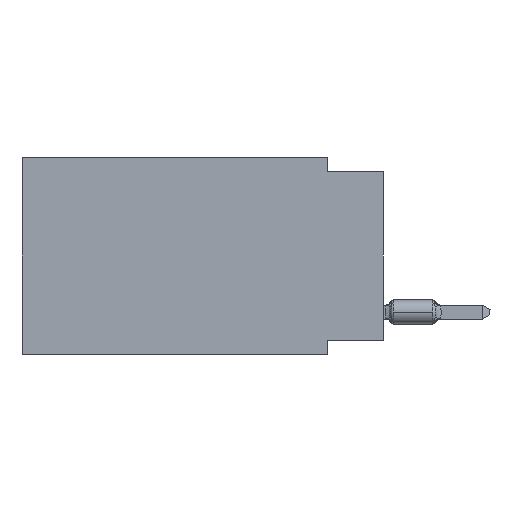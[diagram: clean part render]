
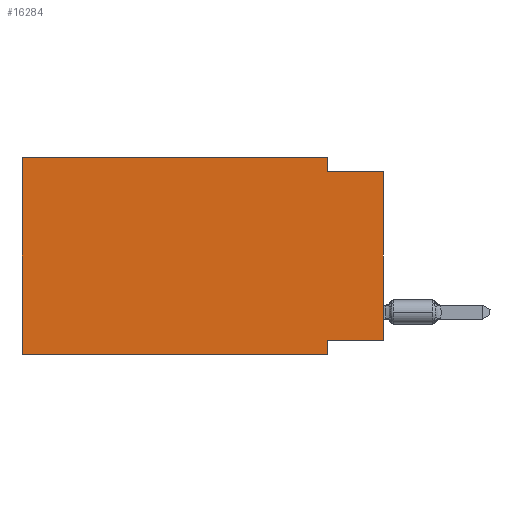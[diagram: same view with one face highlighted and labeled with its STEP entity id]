
A CAD part, left-side view. The second image highlights one B-rep face of the part: STEP entity #16284.
In plain terms, the highlighted planar face has unit normal (-1, 0, 0).
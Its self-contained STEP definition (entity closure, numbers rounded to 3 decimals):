
#670 = ORIENTED_EDGE ( 'NONE', *, *, #5634, .T. ) ;
#1044 = CARTESIAN_POINT ( 'NONE',  ( 0., 0., -0.635 ) ) ;
#1764 = ORIENTED_EDGE ( 'NONE', *, *, #18690, .F. ) ;
#1893 = VERTEX_POINT ( 'NONE', #17982 ) ;
#2091 = DIRECTION ( 'NONE',  ( 0., 0., -1. ) ) ;
#2165 = DIRECTION ( 'NONE',  ( 0., 0., 1. ) ) ;
#3169 = CARTESIAN_POINT ( 'NONE',  ( 0., 2.54, 0. ) ) ;
#3467 = VECTOR ( 'NONE', #2091, 1000. ) ;
#3709 = VERTEX_POINT ( 'NONE', #9611 ) ;
#3777 = AXIS2_PLACEMENT_3D ( 'NONE', #24394, #14852, #5420 ) ;
#3824 = VERTEX_POINT ( 'NONE', #28617 ) ;
#4627 = ORIENTED_EDGE ( 'NONE', *, *, #27068, .F. ) ;
#4704 = DIRECTION ( 'NONE',  ( 0., 0., -1. ) ) ;
#5321 = ORIENTED_EDGE ( 'NONE', *, *, #14407, .T. ) ;
#5398 = ORIENTED_EDGE ( 'NONE', *, *, #9763, .F. ) ;
#5420 = DIRECTION ( 'NONE',  ( 0., 0., -1. ) ) ;
#5634 = EDGE_CURVE ( 'NONE', #28840, #21206, #7386, .T. ) ;
#6299 = CARTESIAN_POINT ( 'NONE',  ( 0., 16.383, 0. ) ) ;
#7386 = LINE ( 'NONE', #14650, #23818 ) ;
#7704 = CARTESIAN_POINT ( 'NONE',  ( 0., 0., -8.255 ) ) ;
#8350 = FACE_OUTER_BOUND ( 'NONE', #13099, .T. ) ;
#9541 = DIRECTION ( 'NONE',  ( 0., -1., 0. ) ) ;
#9611 = CARTESIAN_POINT ( 'NONE',  ( 0., 2.54, -8.89 ) ) ;
#9763 = EDGE_CURVE ( 'NONE', #21178, #3709, #25069, .T. ) ;
#10614 = DIRECTION ( 'NONE',  ( 0., 0., 1. ) ) ;
#11358 = LINE ( 'NONE', #18605, #15515 ) ;
#11413 = DIRECTION ( 'NONE',  ( 0., -1., 0. ) ) ;
#11613 = VECTOR ( 'NONE', #20058, 1000. ) ;
#11984 = CARTESIAN_POINT ( 'NONE',  ( 0., 0., -8.255 ) ) ;
#12189 = LINE ( 'NONE', #7704, #28339 ) ;
#12405 = VECTOR ( 'NONE', #9541, 1000. ) ;
#12839 = PLANE ( 'NONE',  #3777 ) ;
#13099 = EDGE_LOOP ( 'NONE', ( #670, #29649, #20094, #4627, #1764, #5321, #5398, #22240 ) ) ;
#13275 = LINE ( 'NONE', #18043, #11613 ) ;
#13638 = VERTEX_POINT ( 'NONE', #3169 ) ;
#14407 = EDGE_CURVE ( 'NONE', #1893, #3709, #13275, .T. ) ;
#14650 = CARTESIAN_POINT ( 'NONE',  ( 0., 0., 0. ) ) ;
#14852 = DIRECTION ( 'NONE',  ( 1., 0., 0. ) ) ;
#14883 = CARTESIAN_POINT ( 'NONE',  ( 0., 2.54, -0.635 ) ) ;
#14939 = EDGE_CURVE ( 'NONE', #13638, #26555, #11358, .T. ) ;
#15515 = VECTOR ( 'NONE', #4704, 1000. ) ;
#16053 = LINE ( 'NONE', #23612, #12405 ) ;
#16203 = CARTESIAN_POINT ( 'NONE',  ( 0., 16.383, 0. ) ) ;
#16284 = ADVANCED_FACE ( 'NONE', ( #8350 ), #12839, .F. ) ;
#16444 = CARTESIAN_POINT ( 'NONE',  ( 0., 2.54, -8.255 ) ) ;
#16639 = VECTOR ( 'NONE', #11413, 1000. ) ;
#17123 = DIRECTION ( 'NONE',  ( 0., 1., 0. ) ) ;
#17982 = CARTESIAN_POINT ( 'NONE',  ( 0., 16.383, -8.89 ) ) ;
#18043 = CARTESIAN_POINT ( 'NONE',  ( 0., 16.383, -8.89 ) ) ;
#18605 = CARTESIAN_POINT ( 'NONE',  ( 0., 2.54, 0. ) ) ;
#18690 = EDGE_CURVE ( 'NONE', #1893, #3824, #22351, .T. ) ;
#19738 = EDGE_CURVE ( 'NONE', #26555, #21206, #16053, .T. ) ;
#20058 = DIRECTION ( 'NONE',  ( 0., -1., 0. ) ) ;
#20094 = ORIENTED_EDGE ( 'NONE', *, *, #14939, .F. ) ;
#20738 = CARTESIAN_POINT ( 'NONE',  ( 0., 2.54, -8.89 ) ) ;
#20978 = EDGE_CURVE ( 'NONE', #28840, #21178, #12189, .T. ) ;
#21178 = VERTEX_POINT ( 'NONE', #16444 ) ;
#21206 = VERTEX_POINT ( 'NONE', #1044 ) ;
#22240 = ORIENTED_EDGE ( 'NONE', *, *, #20978, .F. ) ;
#22242 = VECTOR ( 'NONE', #10614, 1000. ) ;
#22351 = LINE ( 'NONE', #6299, #22242 ) ;
#23612 = CARTESIAN_POINT ( 'NONE',  ( 0., 0., -0.635 ) ) ;
#23818 = VECTOR ( 'NONE', #2165, 1000. ) ;
#24394 = CARTESIAN_POINT ( 'NONE',  ( 0., 16.383, 0. ) ) ;
#25069 = LINE ( 'NONE', #20738, #3467 ) ;
#26555 = VERTEX_POINT ( 'NONE', #14883 ) ;
#27068 = EDGE_CURVE ( 'NONE', #3824, #13638, #27759, .T. ) ;
#27759 = LINE ( 'NONE', #16203, #16639 ) ;
#28339 = VECTOR ( 'NONE', #17123, 1000. ) ;
#28617 = CARTESIAN_POINT ( 'NONE',  ( 0., 16.383, 0. ) ) ;
#28840 = VERTEX_POINT ( 'NONE', #11984 ) ;
#29649 = ORIENTED_EDGE ( 'NONE', *, *, #19738, .F. ) ;
